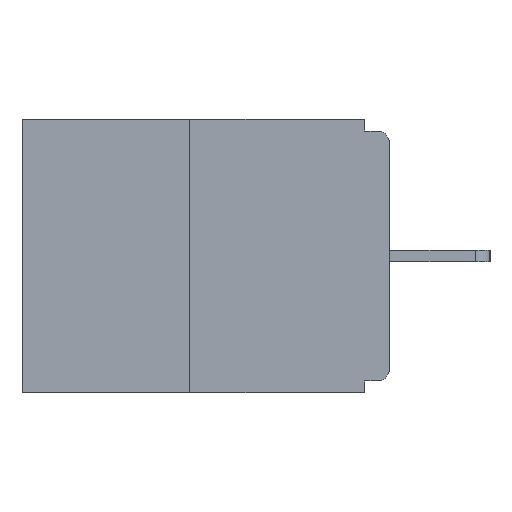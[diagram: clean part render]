
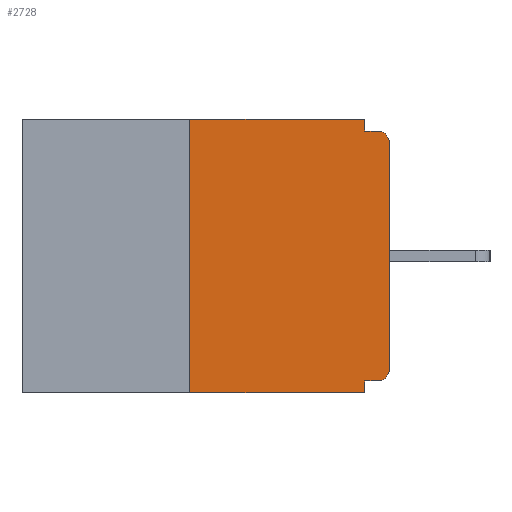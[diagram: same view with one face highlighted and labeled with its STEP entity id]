
A CAD part, left-side view. The second image highlights one B-rep face of the part: STEP entity #2728.
In plain terms, the highlighted planar face has unit normal (-1, 0, 0).
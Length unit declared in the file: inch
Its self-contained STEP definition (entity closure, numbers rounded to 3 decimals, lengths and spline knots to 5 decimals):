
#93 = AXIS2_PLACEMENT_3D ( 'NONE', #8737, #1788, #9915 ) ;
#339 = EDGE_CURVE ( 'NONE', #2374, #3452, #854, .T. ) ;
#439 = AXIS2_PLACEMENT_3D ( 'NONE', #11977, #14748, #5955 ) ;
#675 = CARTESIAN_POINT ( 'NONE',  ( 0., 0., -0.313 ) ) ;
#854 = LINE ( 'NONE', #4435, #6829 ) ;
#864 = CARTESIAN_POINT ( 'NONE',  ( 0., 0.25, -0.343 ) ) ;
#1001 = LINE ( 'NONE', #1549, #3978 ) ;
#1275 = CIRCLE ( 'NONE', #5850, 0.015 ) ;
#1549 = CARTESIAN_POINT ( 'NONE',  ( 0., 0., 0. ) ) ;
#1745 = LINE ( 'NONE', #9292, #13310 ) ;
#1788 = DIRECTION ( 'NONE',  ( -1., 0., 0. ) ) ;
#2164 = EDGE_CURVE ( 'NONE', #6987, #2374, #8857, .T. ) ;
#2374 = VERTEX_POINT ( 'NONE', #14025 ) ;
#2521 = EDGE_CURVE ( 'NONE', #13256, #8335, #14727, .T. ) ;
#2574 = VECTOR ( 'NONE', #4109, 39.37008 ) ;
#2593 = CARTESIAN_POINT ( 'NONE',  ( 0., 0.46, -0.343 ) ) ;
#2728 = ADVANCED_FACE ( 'NONE', ( #10102 ), #13607, .F. ) ;
#3108 = VERTEX_POINT ( 'NONE', #675 ) ;
#3313 = LINE ( 'NONE', #5244, #12015 ) ;
#3399 = CIRCLE ( 'NONE', #93, 0.015 ) ;
#3452 = VERTEX_POINT ( 'NONE', #4047 ) ;
#3540 = CARTESIAN_POINT ( 'NONE',  ( 0., 0.031, -0.343 ) ) ;
#3597 = CARTESIAN_POINT ( 'NONE',  ( 0., 0., -0.328 ) ) ;
#3617 = CARTESIAN_POINT ( 'NONE',  ( 0., 0.031, 0. ) ) ;
#3839 = EDGE_CURVE ( 'NONE', #8335, #10979, #7303, .T. ) ;
#3949 = VECTOR ( 'NONE', #6536, 39.37008 ) ;
#3978 = VECTOR ( 'NONE', #8494, 39.37008 ) ;
#4047 = CARTESIAN_POINT ( 'NONE',  ( 0., 0.015, -0.015 ) ) ;
#4109 = DIRECTION ( 'NONE',  ( 0., 1., 0. ) ) ;
#4248 = ORIENTED_EDGE ( 'NONE', *, *, #2164, .F. ) ;
#4326 = CARTESIAN_POINT ( 'NONE',  ( 0., 0., -0.03 ) ) ;
#4435 = CARTESIAN_POINT ( 'NONE',  ( 0., 0., -0.015 ) ) ;
#4466 = DIRECTION ( 'NONE',  ( 0., -1., 0. ) ) ;
#4738 = CARTESIAN_POINT ( 'NONE',  ( 0., 0.015, -0.313 ) ) ;
#5244 = CARTESIAN_POINT ( 'NONE',  ( 0., 0.25, 0. ) ) ;
#5330 = EDGE_CURVE ( 'NONE', #13724, #6987, #1745, .T. ) ;
#5478 = ORIENTED_EDGE ( 'NONE', *, *, #6855, .F. ) ;
#5825 = CARTESIAN_POINT ( 'NONE',  ( 0., 0.031, 0. ) ) ;
#5850 = AXIS2_PLACEMENT_3D ( 'NONE', #4738, #12674, #5893 ) ;
#5893 = DIRECTION ( 'NONE',  ( 0., 0., -1. ) ) ;
#5955 = DIRECTION ( 'NONE',  ( 0., 0., -1. ) ) ;
#5960 = VERTEX_POINT ( 'NONE', #4326 ) ;
#6123 = EDGE_CURVE ( 'NONE', #9147, #10979, #13823, .T. ) ;
#6245 = VECTOR ( 'NONE', #8037, 39.37008 ) ;
#6536 = DIRECTION ( 'NONE',  ( 0., 0., -1. ) ) ;
#6829 = VECTOR ( 'NONE', #4466, 39.37008 ) ;
#6855 = EDGE_CURVE ( 'NONE', #9147, #13724, #3313, .T. ) ;
#6877 = ORIENTED_EDGE ( 'NONE', *, *, #10103, .T. ) ;
#6987 = VERTEX_POINT ( 'NONE', #5825 ) ;
#7108 = CARTESIAN_POINT ( 'NONE',  ( 0., 0.015, -0.328 ) ) ;
#7303 = LINE ( 'NONE', #3540, #3949 ) ;
#7962 = CARTESIAN_POINT ( 'NONE',  ( 0., 0.031, -0.343 ) ) ;
#8037 = DIRECTION ( 'NONE',  ( 0., 0., -1. ) ) ;
#8335 = VERTEX_POINT ( 'NONE', #14576 ) ;
#8494 = DIRECTION ( 'NONE',  ( 0., 0., 1. ) ) ;
#8737 = CARTESIAN_POINT ( 'NONE',  ( 0., 0.015, -0.03 ) ) ;
#8799 = ORIENTED_EDGE ( 'NONE', *, *, #6123, .T. ) ;
#8857 = LINE ( 'NONE', #3617, #6245 ) ;
#9147 = VERTEX_POINT ( 'NONE', #864 ) ;
#9292 = CARTESIAN_POINT ( 'NONE',  ( 0., 0.46, 0. ) ) ;
#9422 = EDGE_CURVE ( 'NONE', #3108, #5960, #1001, .T. ) ;
#9515 = ORIENTED_EDGE ( 'NONE', *, *, #13155, .T. ) ;
#9553 = DIRECTION ( 'NONE',  ( 0., -1., 0. ) ) ;
#9905 = ORIENTED_EDGE ( 'NONE', *, *, #339, .F. ) ;
#9915 = DIRECTION ( 'NONE',  ( 0., 0., -1. ) ) ;
#10102 = FACE_OUTER_BOUND ( 'NONE', #10761, .T. ) ;
#10103 = EDGE_CURVE ( 'NONE', #5960, #3452, #3399, .T. ) ;
#10761 = EDGE_LOOP ( 'NONE', ( #14176, #5478, #8799, #11839, #14858, #9515, #12562, #6877, #9905, #4248 ) ) ;
#10820 = VECTOR ( 'NONE', #14085, 39.37008 ) ;
#10979 = VERTEX_POINT ( 'NONE', #7962 ) ;
#11839 = ORIENTED_EDGE ( 'NONE', *, *, #3839, .F. ) ;
#11977 = CARTESIAN_POINT ( 'NONE',  ( 0., 0.46, 0. ) ) ;
#12015 = VECTOR ( 'NONE', #12516, 39.37008 ) ;
#12407 = CARTESIAN_POINT ( 'NONE',  ( 0., 0.25, 0. ) ) ;
#12516 = DIRECTION ( 'NONE',  ( 0., 0., 1. ) ) ;
#12562 = ORIENTED_EDGE ( 'NONE', *, *, #9422, .T. ) ;
#12674 = DIRECTION ( 'NONE',  ( -1., 0., 0. ) ) ;
#13155 = EDGE_CURVE ( 'NONE', #13256, #3108, #1275, .T. ) ;
#13256 = VERTEX_POINT ( 'NONE', #7108 ) ;
#13310 = VECTOR ( 'NONE', #9553, 39.37008 ) ;
#13607 = PLANE ( 'NONE',  #439 ) ;
#13724 = VERTEX_POINT ( 'NONE', #12407 ) ;
#13823 = LINE ( 'NONE', #2593, #10820 ) ;
#14025 = CARTESIAN_POINT ( 'NONE',  ( 0., 0.031, -0.015 ) ) ;
#14085 = DIRECTION ( 'NONE',  ( 0., -1., 0. ) ) ;
#14176 = ORIENTED_EDGE ( 'NONE', *, *, #5330, .F. ) ;
#14576 = CARTESIAN_POINT ( 'NONE',  ( 0., 0.031, -0.328 ) ) ;
#14727 = LINE ( 'NONE', #3597, #2574 ) ;
#14748 = DIRECTION ( 'NONE',  ( 1., 0., 0. ) ) ;
#14858 = ORIENTED_EDGE ( 'NONE', *, *, #2521, .F. ) ;
